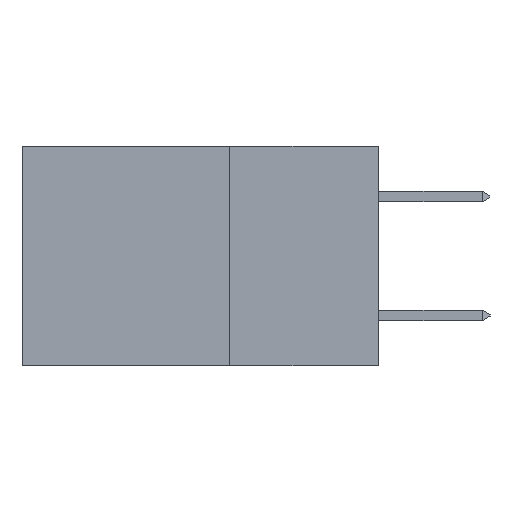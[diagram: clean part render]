
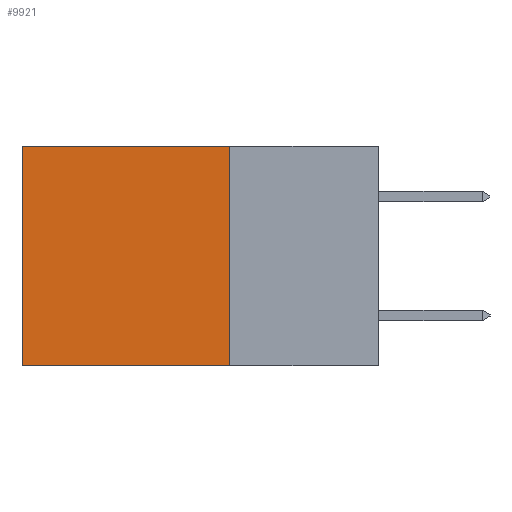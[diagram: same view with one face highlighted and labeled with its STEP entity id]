
A CAD part, left-side view. The second image highlights one B-rep face of the part: STEP entity #9921.
In plain terms, the highlighted planar face has unit normal (-1, 0, 0).
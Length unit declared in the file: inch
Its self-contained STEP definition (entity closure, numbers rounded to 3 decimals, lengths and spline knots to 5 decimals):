
#1370 = PLANE ( 'NONE',  #3933 ) ;
#2694 = CARTESIAN_POINT ( 'NONE',  ( 0.2615, 0.25, 0. ) ) ;
#3616 = LINE ( 'NONE', #17927, #19518 ) ;
#3933 = AXIS2_PLACEMENT_3D ( 'NONE', #12186, #13737, #4485 ) ;
#3985 = DIRECTION ( 'NONE',  ( 0., 0., -1. ) ) ;
#4184 = VECTOR ( 'NONE', #18227, 39.37008 ) ;
#4485 = DIRECTION ( 'NONE',  ( 0., 0., -1. ) ) ;
#5274 = ORIENTED_EDGE ( 'NONE', *, *, #14300, .T. ) ;
#5893 = CARTESIAN_POINT ( 'NONE',  ( 0.2615, 0.6, -0.37 ) ) ;
#5902 = CARTESIAN_POINT ( 'NONE',  ( 0.2615, 0.25, -0.37 ) ) ;
#6821 = ORIENTED_EDGE ( 'NONE', *, *, #12011, .T. ) ;
#6981 = LINE ( 'NONE', #8575, #14244 ) ;
#8575 = CARTESIAN_POINT ( 'NONE',  ( 0.2615, 0.25, -0.37 ) ) ;
#9062 = VERTEX_POINT ( 'NONE', #9991 ) ;
#9106 = EDGE_CURVE ( 'NONE', #12340, #9062, #6981, .T. ) ;
#9473 = VECTOR ( 'NONE', #18244, 39.37008 ) ;
#9659 = VERTEX_POINT ( 'NONE', #14680 ) ;
#9921 = ADVANCED_FACE ( 'NONE', ( #17486 ), #1370, .F. ) ;
#9991 = CARTESIAN_POINT ( 'NONE',  ( 0.2615, 0.25, -0.37 ) ) ;
#10265 = DIRECTION ( 'NONE',  ( 0., 1., 0. ) ) ;
#11142 = ORIENTED_EDGE ( 'NONE', *, *, #9106, .F. ) ;
#12011 = EDGE_CURVE ( 'NONE', #9659, #16670, #13350, .T. ) ;
#12186 = CARTESIAN_POINT ( 'NONE',  ( 0.2615, 0.25, -0.37 ) ) ;
#12340 = VERTEX_POINT ( 'NONE', #2694 ) ;
#13053 = EDGE_CURVE ( 'NONE', #9062, #16670, #18117, .T. ) ;
#13350 = LINE ( 'NONE', #5893, #4184 ) ;
#13737 = DIRECTION ( 'NONE',  ( 1., 0., 0. ) ) ;
#14244 = VECTOR ( 'NONE', #3985, 39.37008 ) ;
#14300 = EDGE_CURVE ( 'NONE', #12340, #9659, #3616, .T. ) ;
#14680 = CARTESIAN_POINT ( 'NONE',  ( 0.2615, 0.6, 0. ) ) ;
#16621 = ORIENTED_EDGE ( 'NONE', *, *, #13053, .F. ) ;
#16670 = VERTEX_POINT ( 'NONE', #17393 ) ;
#17393 = CARTESIAN_POINT ( 'NONE',  ( 0.2615, 0.6, -0.37 ) ) ;
#17486 = FACE_OUTER_BOUND ( 'NONE', #18996, .T. ) ;
#17927 = CARTESIAN_POINT ( 'NONE',  ( 0.2615, 0.25, 0. ) ) ;
#18117 = LINE ( 'NONE', #5902, #9473 ) ;
#18227 = DIRECTION ( 'NONE',  ( 0., 0., -1. ) ) ;
#18244 = DIRECTION ( 'NONE',  ( 0., 1., 0. ) ) ;
#18996 = EDGE_LOOP ( 'NONE', ( #6821, #16621, #11142, #5274 ) ) ;
#19518 = VECTOR ( 'NONE', #10265, 39.37008 ) ;
